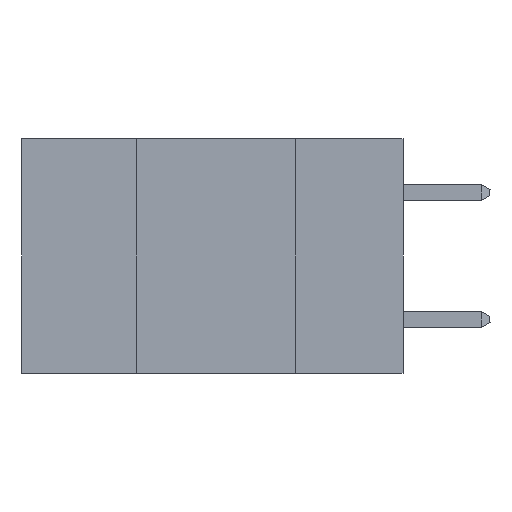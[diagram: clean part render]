
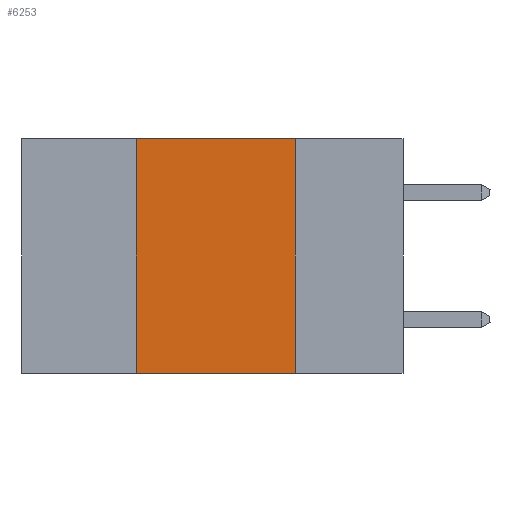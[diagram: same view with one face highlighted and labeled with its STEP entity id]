
A CAD part, left-side view. The second image highlights one B-rep face of the part: STEP entity #6253.
In plain terms, the highlighted planar face has unit normal (-1, 0, 0).
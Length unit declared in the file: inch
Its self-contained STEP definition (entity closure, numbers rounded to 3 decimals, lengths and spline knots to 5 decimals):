
#555 = CARTESIAN_POINT ( 'NONE',  ( 0., 0.6, 0. ) ) ;
#998 = EDGE_LOOP ( 'NONE', ( #23530, #7598, #14167, #21082 ) ) ;
#4616 = LINE ( 'NONE', #555, #23675 ) ;
#6253 = ADVANCED_FACE ( 'NONE', ( #22459 ), #16921, .F. ) ;
#6473 = LINE ( 'NONE', #21397, #20031 ) ;
#7598 = ORIENTED_EDGE ( 'NONE', *, *, #20593, .F. ) ;
#7685 = DIRECTION ( 'NONE',  ( 0., 0., -1. ) ) ;
#7693 = VERTEX_POINT ( 'NONE', #18943 ) ;
#7848 = VERTEX_POINT ( 'NONE', #8439 ) ;
#8108 = DIRECTION ( 'NONE',  ( 0., -1., 0. ) ) ;
#8279 = CARTESIAN_POINT ( 'NONE',  ( 0., 0.42, 0. ) ) ;
#8380 = LINE ( 'NONE', #9565, #13925 ) ;
#8439 = CARTESIAN_POINT ( 'NONE',  ( 0., 0.17, 0. ) ) ;
#8563 = EDGE_CURVE ( 'NONE', #7848, #7693, #6473, .T. ) ;
#9565 = CARTESIAN_POINT ( 'NONE',  ( 0., 0.42, 0. ) ) ;
#9692 = VERTEX_POINT ( 'NONE', #8279 ) ;
#9981 = EDGE_CURVE ( 'NONE', #18426, #7693, #23288, .T. ) ;
#12288 = AXIS2_PLACEMENT_3D ( 'NONE', #16848, #18765, #7685 ) ;
#12973 = VECTOR ( 'NONE', #16778, 39.37008 ) ;
#13925 = VECTOR ( 'NONE', #20572, 39.37008 ) ;
#14025 = EDGE_CURVE ( 'NONE', #18426, #9692, #8380, .T. ) ;
#14167 = ORIENTED_EDGE ( 'NONE', *, *, #14025, .F. ) ;
#16778 = DIRECTION ( 'NONE',  ( 0., -1., 0. ) ) ;
#16848 = CARTESIAN_POINT ( 'NONE',  ( 0., 0.6, 0. ) ) ;
#16921 = PLANE ( 'NONE',  #12288 ) ;
#18426 = VERTEX_POINT ( 'NONE', #18455 ) ;
#18455 = CARTESIAN_POINT ( 'NONE',  ( 0., 0.42, -0.37 ) ) ;
#18765 = DIRECTION ( 'NONE',  ( 1., 0., 0. ) ) ;
#18943 = CARTESIAN_POINT ( 'NONE',  ( 0., 0.17, -0.37 ) ) ;
#20031 = VECTOR ( 'NONE', #21939, 39.37008 ) ;
#20441 = CARTESIAN_POINT ( 'NONE',  ( 0., 0.6, -0.37 ) ) ;
#20572 = DIRECTION ( 'NONE',  ( 0., 0., 1. ) ) ;
#20593 = EDGE_CURVE ( 'NONE', #9692, #7848, #4616, .T. ) ;
#21082 = ORIENTED_EDGE ( 'NONE', *, *, #9981, .T. ) ;
#21397 = CARTESIAN_POINT ( 'NONE',  ( 0., 0.17, 0. ) ) ;
#21939 = DIRECTION ( 'NONE',  ( 0., 0., -1. ) ) ;
#22459 = FACE_OUTER_BOUND ( 'NONE', #998, .T. ) ;
#23288 = LINE ( 'NONE', #20441, #12973 ) ;
#23530 = ORIENTED_EDGE ( 'NONE', *, *, #8563, .F. ) ;
#23675 = VECTOR ( 'NONE', #8108, 39.37008 ) ;
